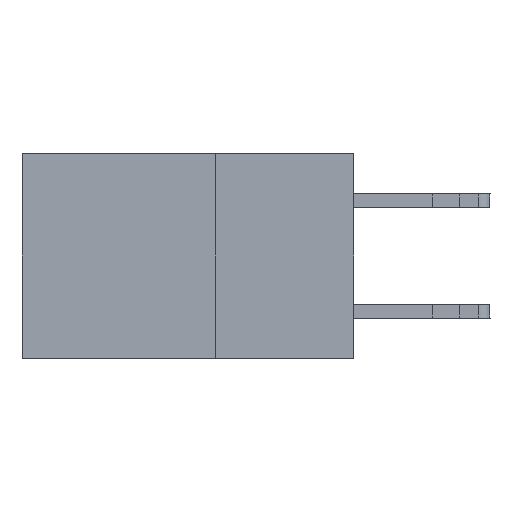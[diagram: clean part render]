
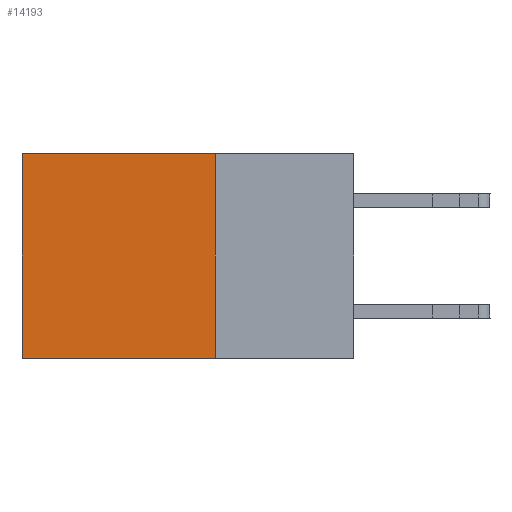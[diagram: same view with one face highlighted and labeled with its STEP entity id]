
A CAD part, left-side view. The second image highlights one B-rep face of the part: STEP entity #14193.
In plain terms, the highlighted planar face has unit normal (-1, 0, 0).
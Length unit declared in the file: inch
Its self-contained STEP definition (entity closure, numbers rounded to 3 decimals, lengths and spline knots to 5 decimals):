
#1351 = EDGE_CURVE ( 'NONE', #9123, #15450, #2014, .T. ) ;
#1426 = LINE ( 'NONE', #18504, #15324 ) ;
#2014 = LINE ( 'NONE', #21250, #2129 ) ;
#2129 = VECTOR ( 'NONE', #7983, 39.37008 ) ;
#2570 = AXIS2_PLACEMENT_3D ( 'NONE', #4650, #26177, #24034 ) ;
#2884 = EDGE_CURVE ( 'NONE', #24795, #15450, #23076, .T. ) ;
#3077 = VERTEX_POINT ( 'NONE', #8102 ) ;
#4650 = CARTESIAN_POINT ( 'NONE',  ( 0.2875, 0.25, 0. ) ) ;
#6677 = EDGE_CURVE ( 'NONE', #3077, #9123, #1426, .T. ) ;
#6781 = ORIENTED_EDGE ( 'NONE', *, *, #2884, .F. ) ;
#7983 = DIRECTION ( 'NONE',  ( 0., 0., -1. ) ) ;
#8102 = CARTESIAN_POINT ( 'NONE',  ( 0.2875, 0.25, 0. ) ) ;
#9123 = VERTEX_POINT ( 'NONE', #10939 ) ;
#9668 = DIRECTION ( 'NONE',  ( 0., 1., 0. ) ) ;
#10939 = CARTESIAN_POINT ( 'NONE',  ( 0.2875, 0.6, 0. ) ) ;
#11507 = VECTOR ( 'NONE', #25589, 39.37008 ) ;
#11650 = ORIENTED_EDGE ( 'NONE', *, *, #1351, .T. ) ;
#12099 = CARTESIAN_POINT ( 'NONE',  ( 0.2875, 0.6, -0.37 ) ) ;
#12749 = ORIENTED_EDGE ( 'NONE', *, *, #6677, .T. ) ;
#14193 = ADVANCED_FACE ( 'NONE', ( #25880 ), #17473, .F. ) ;
#14370 = DIRECTION ( 'NONE',  ( 0., 1., 0. ) ) ;
#15324 = VECTOR ( 'NONE', #9668, 39.37008 ) ;
#15450 = VERTEX_POINT ( 'NONE', #12099 ) ;
#16380 = CARTESIAN_POINT ( 'NONE',  ( 0.2875, 0.25, -0.37 ) ) ;
#17473 = PLANE ( 'NONE',  #2570 ) ;
#18504 = CARTESIAN_POINT ( 'NONE',  ( 0.2875, 0.25, 0. ) ) ;
#19434 = CARTESIAN_POINT ( 'NONE',  ( 0.2875, 0.25, -0.37 ) ) ;
#20589 = EDGE_LOOP ( 'NONE', ( #11650, #6781, #23272, #12749 ) ) ;
#21250 = CARTESIAN_POINT ( 'NONE',  ( 0.2875, 0.6, 0. ) ) ;
#23076 = LINE ( 'NONE', #16380, #26478 ) ;
#23272 = ORIENTED_EDGE ( 'NONE', *, *, #25511, .F. ) ;
#23607 = CARTESIAN_POINT ( 'NONE',  ( 0.2875, 0.25, 0. ) ) ;
#23886 = LINE ( 'NONE', #23607, #11507 ) ;
#24034 = DIRECTION ( 'NONE',  ( 0., 0., -1. ) ) ;
#24795 = VERTEX_POINT ( 'NONE', #19434 ) ;
#25511 = EDGE_CURVE ( 'NONE', #3077, #24795, #23886, .T. ) ;
#25589 = DIRECTION ( 'NONE',  ( 0., 0., -1. ) ) ;
#25880 = FACE_OUTER_BOUND ( 'NONE', #20589, .T. ) ;
#26177 = DIRECTION ( 'NONE',  ( 1., 0., 0. ) ) ;
#26478 = VECTOR ( 'NONE', #14370, 39.37008 ) ;
